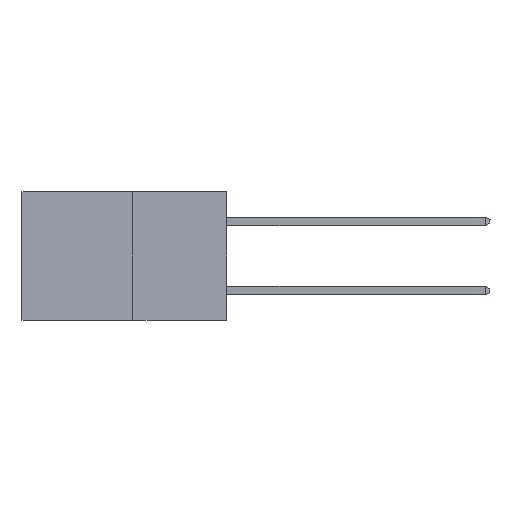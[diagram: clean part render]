
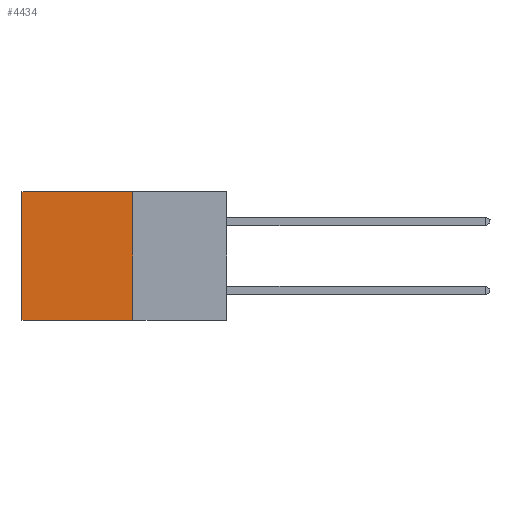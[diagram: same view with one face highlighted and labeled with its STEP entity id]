
A CAD part, left-side view. The second image highlights one B-rep face of the part: STEP entity #4434.
In plain terms, the highlighted planar face has unit normal (-1, 0, 0).
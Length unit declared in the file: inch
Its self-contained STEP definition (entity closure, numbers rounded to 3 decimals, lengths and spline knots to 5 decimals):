
#375 = VERTEX_POINT ( 'NONE', #5778 ) ;
#694 = AXIS2_PLACEMENT_3D ( 'NONE', #3040, #2159, #1679 ) ;
#1084 = VECTOR ( 'NONE', #10296, 39.37008 ) ;
#1246 = ORIENTED_EDGE ( 'NONE', *, *, #5327, .T. ) ;
#1679 = DIRECTION ( 'NONE',  ( 0., 0., -1. ) ) ;
#2068 = VECTOR ( 'NONE', #6485, 39.37008 ) ;
#2159 = DIRECTION ( 'NONE',  ( 1., 0., 0. ) ) ;
#2371 = PLANE ( 'NONE',  #694 ) ;
#2513 = EDGE_CURVE ( 'NONE', #12080, #3864, #9422, .T. ) ;
#2999 = CARTESIAN_POINT ( 'NONE',  ( 0.277, 0.59, -0.37 ) ) ;
#3040 = CARTESIAN_POINT ( 'NONE',  ( 0.277, 0.27, -0.37 ) ) ;
#3540 = LINE ( 'NONE', #12185, #6044 ) ;
#3864 = VERTEX_POINT ( 'NONE', #2999 ) ;
#3885 = LINE ( 'NONE', #7796, #1084 ) ;
#4020 = EDGE_LOOP ( 'NONE', ( #1246, #11370, #4470, #4740 ) ) ;
#4051 = FACE_OUTER_BOUND ( 'NONE', #4020, .T. ) ;
#4161 = EDGE_CURVE ( 'NONE', #375, #5932, #4901, .T. ) ;
#4213 = DIRECTION ( 'NONE',  ( 0., 1., 0. ) ) ;
#4434 = ADVANCED_FACE ( 'NONE', ( #4051 ), #2371, .F. ) ;
#4470 = ORIENTED_EDGE ( 'NONE', *, *, #5819, .F. ) ;
#4740 = ORIENTED_EDGE ( 'NONE', *, *, #4161, .T. ) ;
#4901 = LINE ( 'NONE', #7447, #2068 ) ;
#5327 = EDGE_CURVE ( 'NONE', #5932, #3864, #3885, .T. ) ;
#5778 = CARTESIAN_POINT ( 'NONE',  ( 0.277, 0.27, 0. ) ) ;
#5819 = EDGE_CURVE ( 'NONE', #375, #12080, #3540, .T. ) ;
#5932 = VERTEX_POINT ( 'NONE', #9379 ) ;
#6044 = VECTOR ( 'NONE', #12026, 39.37008 ) ;
#6485 = DIRECTION ( 'NONE',  ( 0., 1., 0. ) ) ;
#6698 = VECTOR ( 'NONE', #4213, 39.37008 ) ;
#7447 = CARTESIAN_POINT ( 'NONE',  ( 0.277, 0.27, 0. ) ) ;
#7796 = CARTESIAN_POINT ( 'NONE',  ( 0.277, 0.59, -0.37 ) ) ;
#9379 = CARTESIAN_POINT ( 'NONE',  ( 0.277, 0.59, 0. ) ) ;
#9422 = LINE ( 'NONE', #9732, #6698 ) ;
#9732 = CARTESIAN_POINT ( 'NONE',  ( 0.277, 0.27, -0.37 ) ) ;
#10296 = DIRECTION ( 'NONE',  ( 0., 0., -1. ) ) ;
#10481 = CARTESIAN_POINT ( 'NONE',  ( 0.277, 0.27, -0.37 ) ) ;
#11370 = ORIENTED_EDGE ( 'NONE', *, *, #2513, .F. ) ;
#12026 = DIRECTION ( 'NONE',  ( 0., 0., -1. ) ) ;
#12080 = VERTEX_POINT ( 'NONE', #10481 ) ;
#12185 = CARTESIAN_POINT ( 'NONE',  ( 0.277, 0.27, -0.37 ) ) ;
